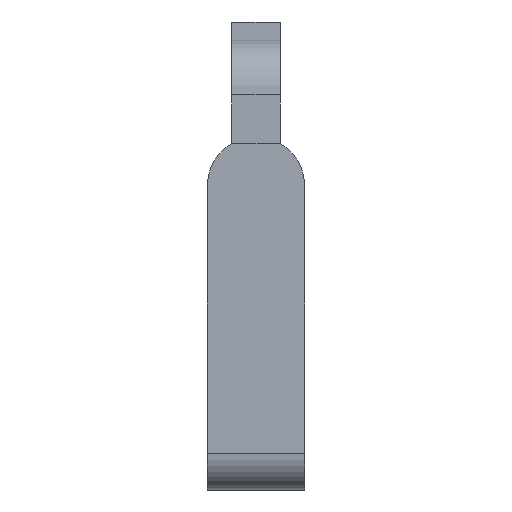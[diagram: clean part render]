
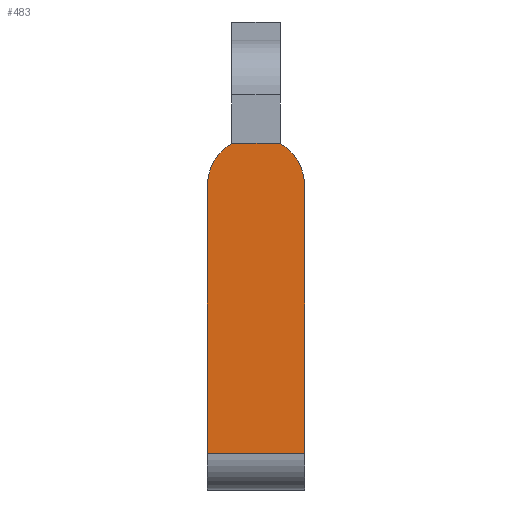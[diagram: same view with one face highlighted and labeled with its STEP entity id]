
A CAD part, left-side view. The second image highlights one B-rep face of the part: STEP entity #483.
In plain terms, the highlighted planar face has unit normal (-1, 0, 0).
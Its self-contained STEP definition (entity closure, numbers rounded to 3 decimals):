
#36 = CARTESIAN_POINT ( 'NONE',  ( 0., 10.16, -28.016 ) ) ;
#100 = CARTESIAN_POINT ( 'NONE',  ( 0., 7.62, 4.399 ) ) ;
#109 = DIRECTION ( 'NONE',  ( 0., 1., 0. ) ) ;
#111 = VERTEX_POINT ( 'NONE', #785 ) ;
#112 = CARTESIAN_POINT ( 'NONE',  ( 0., 5.08, 4.399 ) ) ;
#123 = LINE ( 'NONE', #112, #504 ) ;
#171 = EDGE_CURVE ( 'NONE', #452, #624, #848, .T. ) ;
#183 = VECTOR ( 'NONE', #356, 1000. ) ;
#184 = DIRECTION ( 'NONE',  ( 0., 0., -1. ) ) ;
#188 = DIRECTION ( 'NONE',  ( 1., 0., 0. ) ) ;
#193 = CARTESIAN_POINT ( 'NONE',  ( 0., 5.08, 0. ) ) ;
#240 = CARTESIAN_POINT ( 'NONE',  ( 0., 0., -28.016 ) ) ;
#242 = LINE ( 'NONE', #593, #183 ) ;
#269 = VERTEX_POINT ( 'NONE', #381 ) ;
#294 = VECTOR ( 'NONE', #623, 1000. ) ;
#296 = EDGE_LOOP ( 'NONE', ( #350, #366, #382, #384, #391, #393 ) ) ;
#325 = CARTESIAN_POINT ( 'NONE',  ( 0., 2.54, 4.399 ) ) ;
#338 = DIRECTION ( 'NONE',  ( 0., 0., 1. ) ) ;
#346 = VERTEX_POINT ( 'NONE', #325 ) ;
#350 = ORIENTED_EDGE ( 'NONE', *, *, #390, .F. ) ;
#356 = DIRECTION ( 'NONE',  ( 0., 0., -1. ) ) ;
#366 = ORIENTED_EDGE ( 'NONE', *, *, #418, .T. ) ;
#381 = CARTESIAN_POINT ( 'NONE',  ( 0., 0., 0. ) ) ;
#382 = ORIENTED_EDGE ( 'NONE', *, *, #553, .F. ) ;
#384 = ORIENTED_EDGE ( 'NONE', *, *, #563, .F. ) ;
#390 = EDGE_CURVE ( 'NONE', #346, #269, #551, .T. ) ;
#391 = ORIENTED_EDGE ( 'NONE', *, *, #171, .F. ) ;
#393 = ORIENTED_EDGE ( 'NONE', *, *, #698, .F. ) ;
#395 = AXIS2_PLACEMENT_3D ( 'NONE', #193, #188, #184 ) ;
#418 = EDGE_CURVE ( 'NONE', #346, #562, #123, .T. ) ;
#431 = VECTOR ( 'NONE', #338, 1000. ) ;
#452 = VERTEX_POINT ( 'NONE', #240 ) ;
#483 = ADVANCED_FACE ( 'NONE', ( #801 ), #582, .F. ) ;
#494 = DIRECTION ( 'NONE',  ( 0., 0., -1. ) ) ;
#498 = LINE ( 'NONE', #36, #431 ) ;
#504 = VECTOR ( 'NONE', #109, 1000. ) ;
#547 = DIRECTION ( 'NONE',  ( 0., 0., -1. ) ) ;
#550 = DIRECTION ( 'NONE',  ( 1., 0., 0. ) ) ;
#551 = CIRCLE ( 'NONE', #395, 5.08 ) ;
#553 = EDGE_CURVE ( 'NONE', #111, #562, #763, .T. ) ;
#562 = VERTEX_POINT ( 'NONE', #100 ) ;
#563 = EDGE_CURVE ( 'NONE', #624, #111, #498, .T. ) ;
#580 = DIRECTION ( 'NONE',  ( 1., 0., 0. ) ) ;
#581 = CARTESIAN_POINT ( 'NONE',  ( 0., 0., -28.016 ) ) ;
#582 = PLANE ( 'NONE',  #713 ) ;
#593 = CARTESIAN_POINT ( 'NONE',  ( 0., 0., 0. ) ) ;
#604 = CARTESIAN_POINT ( 'NONE',  ( 0., 5.08, 0. ) ) ;
#623 = DIRECTION ( 'NONE',  ( 0., 1., 0. ) ) ;
#624 = VERTEX_POINT ( 'NONE', #756 ) ;
#682 = AXIS2_PLACEMENT_3D ( 'NONE', #846, #550, #494 ) ;
#698 = EDGE_CURVE ( 'NONE', #269, #452, #242, .T. ) ;
#713 = AXIS2_PLACEMENT_3D ( 'NONE', #604, #580, #547 ) ;
#756 = CARTESIAN_POINT ( 'NONE',  ( 0., 10.16, -28.016 ) ) ;
#763 = CIRCLE ( 'NONE', #682, 5.08 ) ;
#785 = CARTESIAN_POINT ( 'NONE',  ( 0., 10.16, 0. ) ) ;
#801 = FACE_OUTER_BOUND ( 'NONE', #296, .T. ) ;
#846 = CARTESIAN_POINT ( 'NONE',  ( 0., 5.08, 0. ) ) ;
#848 = LINE ( 'NONE', #581, #294 ) ;
